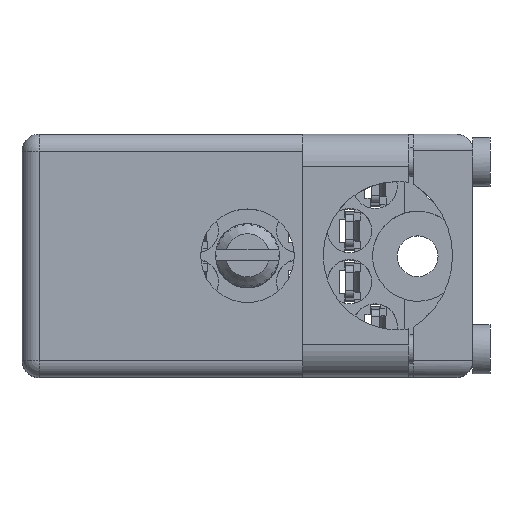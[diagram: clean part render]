
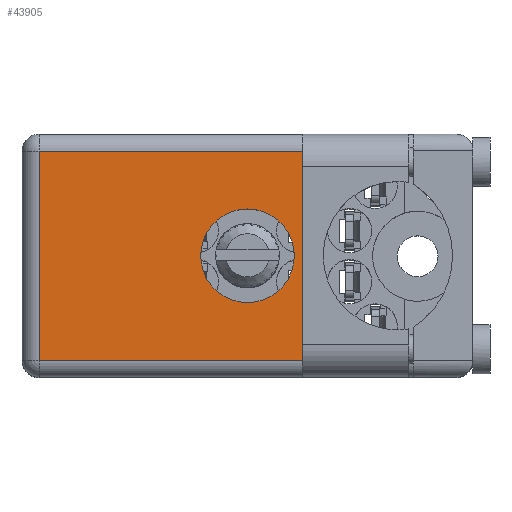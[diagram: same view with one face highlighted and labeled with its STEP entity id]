
A CAD part, top view. The second image highlights one B-rep face of the part: STEP entity #43905.
In plain terms, the highlighted face is planar.
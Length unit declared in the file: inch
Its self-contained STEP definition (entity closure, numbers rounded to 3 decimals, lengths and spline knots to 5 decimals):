
#99 = CARTESIAN_POINT ( 'NONE',  ( 0.05, 0.906, -0.665 ) ) ;
#1082 = EDGE_CURVE ( 'NONE', #24358, #163006, #67061, .T. ) ;
#4780 = DIRECTION ( 'NONE',  ( 0., 0., 1. ) ) ;
#5198 = ORIENTED_EDGE ( 'NONE', *, *, #36021, .F. ) ;
#5299 = VECTOR ( 'NONE', #168342, 39.37008 ) ;
#5582 = VECTOR ( 'NONE', #110831, 39.37008 ) ;
#6353 = CARTESIAN_POINT ( 'NONE',  ( 0.865, 0.906, -0.6025 ) ) ;
#7157 = VECTOR ( 'NONE', #92535, 39.37008 ) ;
#8124 = CARTESIAN_POINT ( 'NONE',  ( 1.15, 0.906, -0.665 ) ) ;
#17772 = VERTEX_POINT ( 'NONE', #6353 ) ;
#19265 = CARTESIAN_POINT ( 'NONE',  ( 0., 0.906, -0.715 ) ) ;
#20922 = LINE ( 'NONE', #27926, #108250 ) ;
#24358 = VERTEX_POINT ( 'NONE', #111849 ) ;
#27921 = LINE ( 'NONE', #62488, #7157 ) ;
#27926 = CARTESIAN_POINT ( 'NONE',  ( 0., 0.906, -0.665 ) ) ;
#28059 = VECTOR ( 'NONE', #143732, 39.37008 ) ;
#31608 = VERTEX_POINT ( 'NONE', #94361 ) ;
#31808 = ORIENTED_EDGE ( 'NONE', *, *, #1082, .T. ) ;
#34791 = ORIENTED_EDGE ( 'NONE', *, *, #181657, .T. ) ;
#36021 = EDGE_CURVE ( 'NONE', #146184, #31608, #93487, .T. ) ;
#39077 = CARTESIAN_POINT ( 'NONE',  ( 1.15, 0.906, -0.1125 ) ) ;
#39448 = ORIENTED_EDGE ( 'NONE', *, *, #182223, .F. ) ;
#39507 = FACE_BOUND ( 'NONE', #84148, .T. ) ;
#41730 = FACE_OUTER_BOUND ( 'NONE', #76655, .T. ) ;
#43905 = ADVANCED_FACE ( 'NONE', ( #41730, #39507 ), #136608, .T. ) ;
#45930 = DIRECTION ( 'NONE',  ( 0., 1., 0. ) ) ;
#48907 = DIRECTION ( 'NONE',  ( 0., 1., 0. ) ) ;
#50562 = CARTESIAN_POINT ( 'NONE',  ( 1.15, 0.906, -0.715 ) ) ;
#55800 = CARTESIAN_POINT ( 'NONE',  ( 1.15, 0.906, -0.05 ) ) ;
#56239 = LINE ( 'NONE', #124847, #5582 ) ;
#56891 = DIRECTION ( 'NONE',  ( 0., 1., 0. ) ) ;
#61937 = CARTESIAN_POINT ( 'NONE',  ( 0.865, 0.906, -0.1125 ) ) ;
#62488 = CARTESIAN_POINT ( 'NONE',  ( 0.865, 0.906, -0.1125 ) ) ;
#66453 = CARTESIAN_POINT ( 'NONE',  ( 0.865, 0.906, -0.6025 ) ) ;
#67061 = LINE ( 'NONE', #70078, #28059 ) ;
#68477 = CARTESIAN_POINT ( 'NONE',  ( 1.15, 0.906, -0.6025 ) ) ;
#70078 = CARTESIAN_POINT ( 'NONE',  ( 1.15, 0.906, -0.05 ) ) ;
#71559 = CARTESIAN_POINT ( 'NONE',  ( 0.6625, 0.906, -0.3575 ) ) ;
#76655 = EDGE_LOOP ( 'NONE', ( #34791, #31808, #170896, #115470, #117975, #174117, #39448, #132350 ) ) ;
#77205 = LINE ( 'NONE', #50562, #111701 ) ;
#77336 = VECTOR ( 'NONE', #148366, 39.37008 ) ;
#77382 = CARTESIAN_POINT ( 'NONE',  ( 1.15, 0.906, -0.715 ) ) ;
#80422 = AXIS2_PLACEMENT_3D ( 'NONE', #71559, #56891, #87517 ) ;
#80531 = DIRECTION ( 'NONE',  ( 0., 0., 1. ) ) ;
#81183 = LINE ( 'NONE', #66453, #5299 ) ;
#82690 = VERTEX_POINT ( 'NONE', #8124 ) ;
#84148 = EDGE_LOOP ( 'NONE', ( #5198, #141688 ) ) ;
#87517 = DIRECTION ( 'NONE',  ( 0., 0., 1. ) ) ;
#87971 = EDGE_CURVE ( 'NONE', #82690, #138409, #20922, .T. ) ;
#89474 = CARTESIAN_POINT ( 'NONE',  ( 0.6625, 0.906, -0.3575 ) ) ;
#92535 = DIRECTION ( 'NONE',  ( 0., 0., -1. ) ) ;
#93487 = CIRCLE ( 'NONE', #105977, 0.1375 ) ;
#94361 = CARTESIAN_POINT ( 'NONE',  ( 0.6625, 0.906, -0.495 ) ) ;
#105977 = AXIS2_PLACEMENT_3D ( 'NONE', #89474, #45930, #117149 ) ;
#108250 = VECTOR ( 'NONE', #157447, 39.37008 ) ;
#110831 = DIRECTION ( 'NONE',  ( 0., 0., 1. ) ) ;
#111208 = VECTOR ( 'NONE', #4780, 39.37008 ) ;
#111701 = VECTOR ( 'NONE', #80531, 39.37008 ) ;
#111849 = CARTESIAN_POINT ( 'NONE',  ( 0.05, 0.906, -0.05 ) ) ;
#115470 = ORIENTED_EDGE ( 'NONE', *, *, #115775, .T. ) ;
#115775 = EDGE_CURVE ( 'NONE', #164997, #127946, #120918, .T. ) ;
#117149 = DIRECTION ( 'NONE',  ( 0., 0., 1. ) ) ;
#117975 = ORIENTED_EDGE ( 'NONE', *, *, #155943, .T. ) ;
#119713 = EDGE_CURVE ( 'NONE', #17772, #179872, #81183, .T. ) ;
#120918 = LINE ( 'NONE', #61937, #77336 ) ;
#122682 = LINE ( 'NONE', #77382, #111208 ) ;
#124847 = CARTESIAN_POINT ( 'NONE',  ( 0.05, 0.906, -0.715 ) ) ;
#127946 = VERTEX_POINT ( 'NONE', #173296 ) ;
#132350 = ORIENTED_EDGE ( 'NONE', *, *, #87971, .T. ) ;
#134504 = EDGE_CURVE ( 'NONE', #164997, #163006, #77205, .T. ) ;
#136608 = PLANE ( 'NONE',  #165930 ) ;
#138409 = VERTEX_POINT ( 'NONE', #99 ) ;
#141688 = ORIENTED_EDGE ( 'NONE', *, *, #155681, .F. ) ;
#143732 = DIRECTION ( 'NONE',  ( 1., 0., 0. ) ) ;
#145037 = CIRCLE ( 'NONE', #80422, 0.1375 ) ;
#146184 = VERTEX_POINT ( 'NONE', #183304 ) ;
#148366 = DIRECTION ( 'NONE',  ( -1., 0., 0. ) ) ;
#151350 = DIRECTION ( 'NONE',  ( 0., 0., 1. ) ) ;
#155681 = EDGE_CURVE ( 'NONE', #31608, #146184, #145037, .T. ) ;
#155943 = EDGE_CURVE ( 'NONE', #127946, #17772, #27921, .T. ) ;
#157447 = DIRECTION ( 'NONE',  ( -1., 0., 0. ) ) ;
#163006 = VERTEX_POINT ( 'NONE', #55800 ) ;
#164997 = VERTEX_POINT ( 'NONE', #39077 ) ;
#165930 = AXIS2_PLACEMENT_3D ( 'NONE', #19265, #48907, #151350 ) ;
#168342 = DIRECTION ( 'NONE',  ( 1., 0., 0. ) ) ;
#170896 = ORIENTED_EDGE ( 'NONE', *, *, #134504, .F. ) ;
#173296 = CARTESIAN_POINT ( 'NONE',  ( 0.865, 0.906, -0.1125 ) ) ;
#174117 = ORIENTED_EDGE ( 'NONE', *, *, #119713, .T. ) ;
#179872 = VERTEX_POINT ( 'NONE', #68477 ) ;
#181657 = EDGE_CURVE ( 'NONE', #138409, #24358, #56239, .T. ) ;
#182223 = EDGE_CURVE ( 'NONE', #82690, #179872, #122682, .T. ) ;
#183304 = CARTESIAN_POINT ( 'NONE',  ( 0.6625, 0.906, -0.22 ) ) ;
